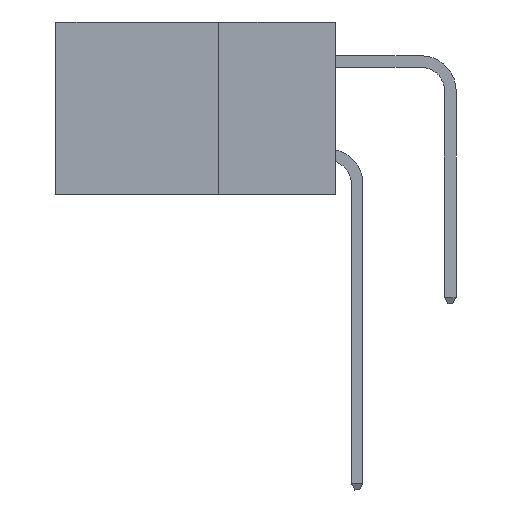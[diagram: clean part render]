
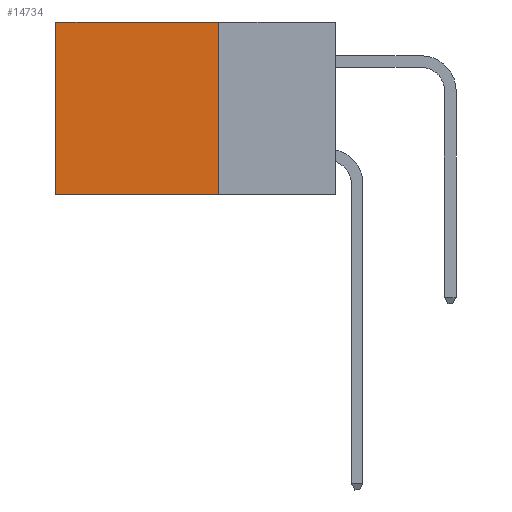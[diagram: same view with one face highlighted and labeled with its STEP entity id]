
A CAD part, left-side view. The second image highlights one B-rep face of the part: STEP entity #14734.
In plain terms, the highlighted planar face has unit normal (-1, 0, 0).
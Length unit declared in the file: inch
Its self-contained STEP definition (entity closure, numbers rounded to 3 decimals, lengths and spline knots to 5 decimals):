
#514 = CARTESIAN_POINT ( 'NONE',  ( 0.2875, 0.6, 0. ) ) ;
#581 = CARTESIAN_POINT ( 'NONE',  ( 0.2875, 0.25, 0. ) ) ;
#1337 = CARTESIAN_POINT ( 'NONE',  ( 0.2875, 0.25, 0. ) ) ;
#1694 = DIRECTION ( 'NONE',  ( 0., 1., 0. ) ) ;
#2056 = EDGE_LOOP ( 'NONE', ( #16118, #6572, #10824, #10957 ) ) ;
#2774 = CARTESIAN_POINT ( 'NONE',  ( 0.2875, 0.25, 0. ) ) ;
#3731 = VERTEX_POINT ( 'NONE', #13708 ) ;
#3881 = DIRECTION ( 'NONE',  ( 0., 0., -1. ) ) ;
#4184 = DIRECTION ( 'NONE',  ( 0., 0., -1. ) ) ;
#4781 = CARTESIAN_POINT ( 'NONE',  ( 0.2875, 0.25, 0. ) ) ;
#5441 = EDGE_CURVE ( 'NONE', #12006, #9690, #17112, .T. ) ;
#6370 = VECTOR ( 'NONE', #12334, 39.37008 ) ;
#6511 = CARTESIAN_POINT ( 'NONE',  ( 0.2875, 0.6, 0. ) ) ;
#6535 = EDGE_CURVE ( 'NONE', #9690, #13427, #16848, .T. ) ;
#6572 = ORIENTED_EDGE ( 'NONE', *, *, #8603, .F. ) ;
#7150 = AXIS2_PLACEMENT_3D ( 'NONE', #2774, #12367, #4184 ) ;
#8603 = EDGE_CURVE ( 'NONE', #3731, #13427, #13519, .T. ) ;
#9538 = VECTOR ( 'NONE', #1694, 39.37008 ) ;
#9690 = VERTEX_POINT ( 'NONE', #6511 ) ;
#10824 = ORIENTED_EDGE ( 'NONE', *, *, #11167, .F. ) ;
#10957 = ORIENTED_EDGE ( 'NONE', *, *, #5441, .T. ) ;
#10993 = CARTESIAN_POINT ( 'NONE',  ( 0.2875, 0.25, -0.37 ) ) ;
#11023 = PLANE ( 'NONE',  #7150 ) ;
#11167 = EDGE_CURVE ( 'NONE', #12006, #3731, #16791, .T. ) ;
#12006 = VERTEX_POINT ( 'NONE', #581 ) ;
#12334 = DIRECTION ( 'NONE',  ( 0., 1., 0. ) ) ;
#12361 = DIRECTION ( 'NONE',  ( 0., 0., -1. ) ) ;
#12367 = DIRECTION ( 'NONE',  ( 1., 0., 0. ) ) ;
#12819 = VECTOR ( 'NONE', #12361, 39.37008 ) ;
#13090 = FACE_OUTER_BOUND ( 'NONE', #2056, .T. ) ;
#13282 = VECTOR ( 'NONE', #3881, 39.37008 ) ;
#13427 = VERTEX_POINT ( 'NONE', #15953 ) ;
#13519 = LINE ( 'NONE', #10993, #6370 ) ;
#13708 = CARTESIAN_POINT ( 'NONE',  ( 0.2875, 0.25, -0.37 ) ) ;
#14734 = ADVANCED_FACE ( 'NONE', ( #13090 ), #11023, .F. ) ;
#15953 = CARTESIAN_POINT ( 'NONE',  ( 0.2875, 0.6, -0.37 ) ) ;
#16118 = ORIENTED_EDGE ( 'NONE', *, *, #6535, .T. ) ;
#16791 = LINE ( 'NONE', #1337, #12819 ) ;
#16848 = LINE ( 'NONE', #514, #13282 ) ;
#17112 = LINE ( 'NONE', #4781, #9538 ) ;
